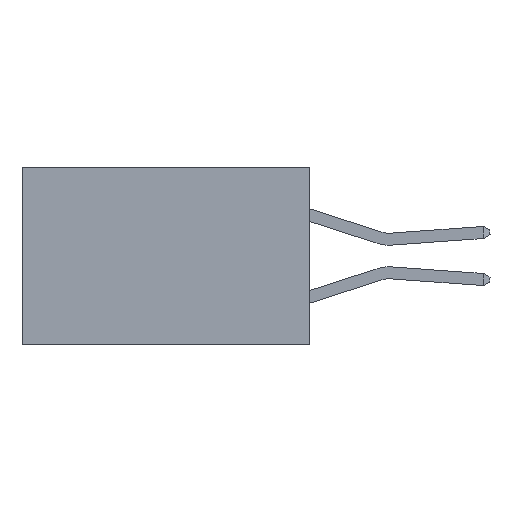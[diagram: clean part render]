
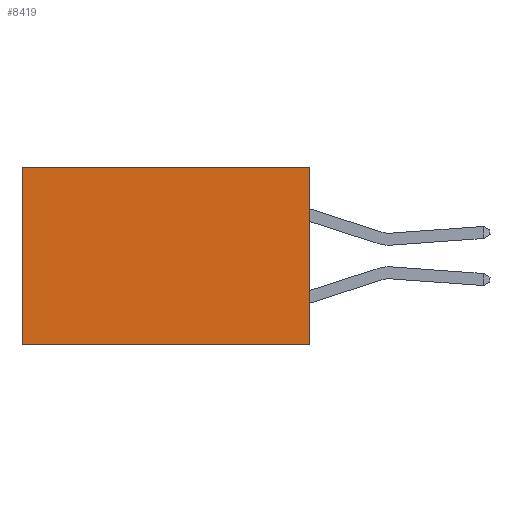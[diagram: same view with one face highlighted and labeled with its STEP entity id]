
A CAD part, left-side view. The second image highlights one B-rep face of the part: STEP entity #8419.
In plain terms, the highlighted planar face has unit normal (-1, 0, 0).
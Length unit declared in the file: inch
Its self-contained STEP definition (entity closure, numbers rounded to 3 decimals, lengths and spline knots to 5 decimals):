
#20 = CARTESIAN_POINT ( 'NONE',  ( 0.2615, 0., 0. ) ) ;
#268 = DIRECTION ( 'NONE',  ( 0., 1., 0. ) ) ;
#306 = CARTESIAN_POINT ( 'NONE',  ( 0.2615, 0., -0.37 ) ) ;
#1184 = ORIENTED_EDGE ( 'NONE', *, *, #9035, .F. ) ;
#1728 = ORIENTED_EDGE ( 'NONE', *, *, #9999, .T. ) ;
#1900 = CARTESIAN_POINT ( 'NONE',  ( 0.2615, 0., -0.37 ) ) ;
#3007 = VERTEX_POINT ( 'NONE', #11153 ) ;
#3085 = CARTESIAN_POINT ( 'NONE',  ( 0.2615, 0.6, -0.37 ) ) ;
#3237 = LINE ( 'NONE', #7674, #7891 ) ;
#3547 = LINE ( 'NONE', #10267, #5549 ) ;
#3746 = EDGE_LOOP ( 'NONE', ( #8405, #10808, #1184, #1728 ) ) ;
#3890 = LINE ( 'NONE', #306, #8266 ) ;
#4459 = AXIS2_PLACEMENT_3D ( 'NONE', #5625, #5510, #5459 ) ;
#4686 = EDGE_CURVE ( 'NONE', #3007, #6653, #3237, .T. ) ;
#5252 = CARTESIAN_POINT ( 'NONE',  ( 0.2615, 0., 0. ) ) ;
#5423 = DIRECTION ( 'NONE',  ( 0., 1., 0. ) ) ;
#5459 = DIRECTION ( 'NONE',  ( 0., 0., -1. ) ) ;
#5510 = DIRECTION ( 'NONE',  ( 1., 0., 0. ) ) ;
#5549 = VECTOR ( 'NONE', #10198, 39.37008 ) ;
#5622 = PLANE ( 'NONE',  #4459 ) ;
#5625 = CARTESIAN_POINT ( 'NONE',  ( 0.2615, 0., -0.37 ) ) ;
#6548 = VERTEX_POINT ( 'NONE', #20 ) ;
#6653 = VERTEX_POINT ( 'NONE', #3085 ) ;
#7674 = CARTESIAN_POINT ( 'NONE',  ( 0.2615, 0.6, -0.37 ) ) ;
#7891 = VECTOR ( 'NONE', #9882, 39.37008 ) ;
#8266 = VECTOR ( 'NONE', #268, 39.37008 ) ;
#8405 = ORIENTED_EDGE ( 'NONE', *, *, #4686, .T. ) ;
#8419 = ADVANCED_FACE ( 'NONE', ( #9803 ), #5622, .F. ) ;
#8670 = VERTEX_POINT ( 'NONE', #1900 ) ;
#8834 = LINE ( 'NONE', #5252, #9105 ) ;
#9035 = EDGE_CURVE ( 'NONE', #6548, #8670, #3547, .T. ) ;
#9105 = VECTOR ( 'NONE', #5423, 39.37008 ) ;
#9803 = FACE_OUTER_BOUND ( 'NONE', #3746, .T. ) ;
#9882 = DIRECTION ( 'NONE',  ( 0., 0., -1. ) ) ;
#9999 = EDGE_CURVE ( 'NONE', #6548, #3007, #8834, .T. ) ;
#10198 = DIRECTION ( 'NONE',  ( 0., 0., -1. ) ) ;
#10267 = CARTESIAN_POINT ( 'NONE',  ( 0.2615, 0., -0.37 ) ) ;
#10808 = ORIENTED_EDGE ( 'NONE', *, *, #10919, .F. ) ;
#10919 = EDGE_CURVE ( 'NONE', #8670, #6653, #3890, .T. ) ;
#11153 = CARTESIAN_POINT ( 'NONE',  ( 0.2615, 0.6, 0. ) ) ;
